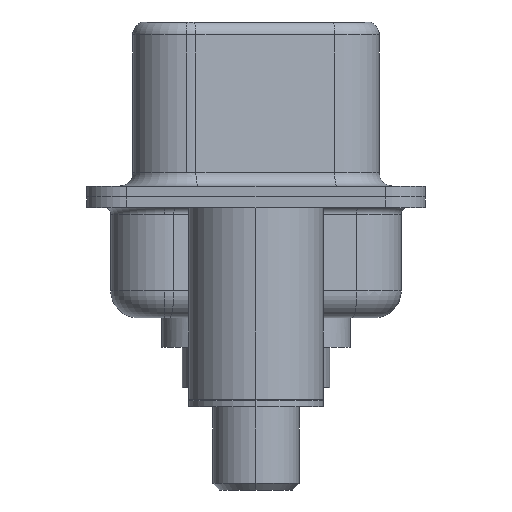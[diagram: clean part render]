
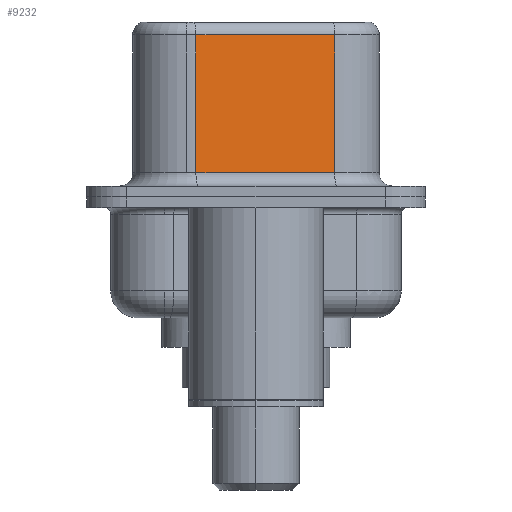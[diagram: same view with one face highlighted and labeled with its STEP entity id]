
A CAD part, left-side view. The second image highlights one B-rep face of the part: STEP entity #9232.
In plain terms, the highlighted planar face has unit normal (-0.985, -0.174, 0).
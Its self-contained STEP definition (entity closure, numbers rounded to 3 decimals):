
#337 = ORIENTED_EDGE ( 'NONE', *, *, #4664, .F. ) ;
#600 = CARTESIAN_POINT ( 'NONE',  ( 4.58, -2.927, 0.9 ) ) ;
#1205 = VECTOR ( 'NONE', #1263, 1000. ) ;
#1263 = DIRECTION ( 'NONE',  ( -0.174, 0.985, 0. ) ) ;
#1417 = CARTESIAN_POINT ( 'NONE',  ( 3.67, 2.233, 0.9 ) ) ;
#2088 = LINE ( 'NONE', #3068, #8165 ) ;
#2219 = VERTEX_POINT ( 'NONE', #9508 ) ;
#3068 = CARTESIAN_POINT ( 'NONE',  ( 4.58, -2.927, 0.9 ) ) ;
#4342 = LINE ( 'NONE', #8120, #1205 ) ;
#4462 = VERTEX_POINT ( 'NONE', #9876 ) ;
#4587 = FACE_OUTER_BOUND ( 'NONE', #11738, .T. ) ;
#4664 = EDGE_CURVE ( 'NONE', #4462, #11980, #12975, .T. ) ;
#5421 = DIRECTION ( 'NONE',  ( -0.174, 0.985, 0. ) ) ;
#5937 = DIRECTION ( 'NONE',  ( 0.985, 0.174, 0. ) ) ;
#6112 = AXIS2_PLACEMENT_3D ( 'NONE', #6145, #5937, #5421 ) ;
#6145 = CARTESIAN_POINT ( 'NONE',  ( 4.58, -2.927, 6.52 ) ) ;
#6744 = PLANE ( 'NONE',  #6112 ) ;
#7668 = DIRECTION ( 'NONE',  ( 0.174, -0.985, 0. ) ) ;
#8120 = CARTESIAN_POINT ( 'NONE',  ( 4.58, -2.927, 6.02 ) ) ;
#8135 = CARTESIAN_POINT ( 'NONE',  ( 3.67, 2.233, 6.52 ) ) ;
#8165 = VECTOR ( 'NONE', #7668, 1000. ) ;
#8502 = ORIENTED_EDGE ( 'NONE', *, *, #12469, .T. ) ;
#9232 = ADVANCED_FACE ( 'NONE', ( #4587 ), #6744, .F. ) ;
#9235 = DIRECTION ( 'NONE',  ( 0., 0., -1. ) ) ;
#9434 = CARTESIAN_POINT ( 'NONE',  ( 4.58, -2.927, 6.52 ) ) ;
#9508 = CARTESIAN_POINT ( 'NONE',  ( 3.67, 2.233, 6.02 ) ) ;
#9876 = CARTESIAN_POINT ( 'NONE',  ( 4.58, -2.927, 6.02 ) ) ;
#9899 = VECTOR ( 'NONE', #10525, 1000. ) ;
#10519 = ORIENTED_EDGE ( 'NONE', *, *, #14814, .T. ) ;
#10525 = DIRECTION ( 'NONE',  ( 0., 0., -1. ) ) ;
#11679 = LINE ( 'NONE', #8135, #12039 ) ;
#11738 = EDGE_LOOP ( 'NONE', ( #337, #8502, #13675, #10519 ) ) ;
#11766 = VERTEX_POINT ( 'NONE', #1417 ) ;
#11980 = VERTEX_POINT ( 'NONE', #600 ) ;
#12039 = VECTOR ( 'NONE', #9235, 1000. ) ;
#12469 = EDGE_CURVE ( 'NONE', #4462, #2219, #4342, .T. ) ;
#12975 = LINE ( 'NONE', #9434, #9899 ) ;
#13675 = ORIENTED_EDGE ( 'NONE', *, *, #14455, .T. ) ;
#14455 = EDGE_CURVE ( 'NONE', #2219, #11766, #11679, .T. ) ;
#14814 = EDGE_CURVE ( 'NONE', #11766, #11980, #2088, .T. ) ;
